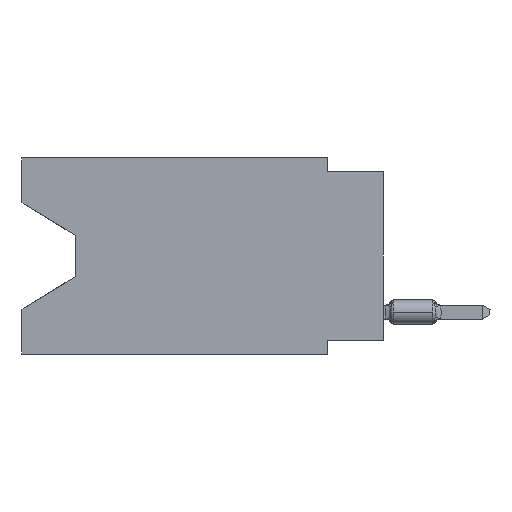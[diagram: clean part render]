
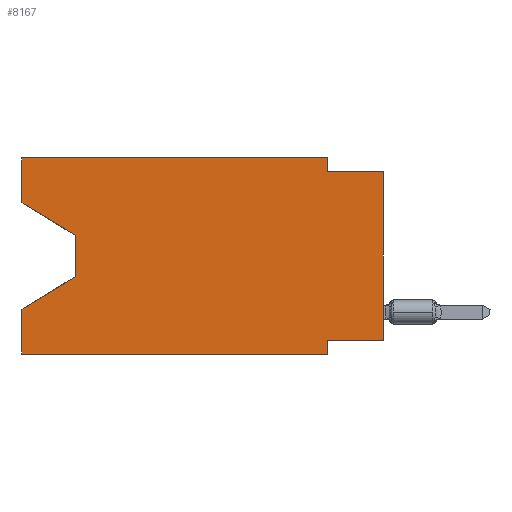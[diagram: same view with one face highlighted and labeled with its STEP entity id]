
A CAD part, left-side view. The second image highlights one B-rep face of the part: STEP entity #8167.
In plain terms, the highlighted planar face has unit normal (-1, 0, 0).
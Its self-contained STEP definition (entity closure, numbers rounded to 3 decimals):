
#788 = DIRECTION ( 'NONE',  ( 0., -1., 0. ) ) ;
#833 = VECTOR ( 'NONE', #54040, 1000. ) ;
#1441 = ORIENTED_EDGE ( 'NONE', *, *, #10999, .F. ) ;
#1702 = ORIENTED_EDGE ( 'NONE', *, *, #21773, .T. ) ;
#2384 = VERTEX_POINT ( 'NONE', #18390 ) ;
#2740 = EDGE_LOOP ( 'NONE', ( #49282, #25133, #4400, #50572, #1702, #9972, #33076, #35058, #36360, #19335, #1441, #18348 ) ) ;
#3293 = VECTOR ( 'NONE', #17079, 1000. ) ;
#3613 = AXIS2_PLACEMENT_3D ( 'NONE', #37514, #12886, #21559 ) ;
#4103 = EDGE_CURVE ( 'NONE', #17922, #8524, #13659, .T. ) ;
#4398 = EDGE_CURVE ( 'NONE', #19168, #21981, #38615, .T. ) ;
#4400 = ORIENTED_EDGE ( 'NONE', *, *, #4398, .T. ) ;
#4711 = LINE ( 'NONE', #21198, #5902 ) ;
#5011 = LINE ( 'NONE', #39121, #32295 ) ;
#5902 = VECTOR ( 'NONE', #788, 1000. ) ;
#5940 = LINE ( 'NONE', #22972, #15642 ) ;
#6770 = DIRECTION ( 'NONE',  ( 0., 0., 1. ) ) ;
#7312 = CARTESIAN_POINT ( 'NONE',  ( 0., 0., -0.635 ) ) ;
#7810 = CARTESIAN_POINT ( 'NONE',  ( 0., 2.54, -8.255 ) ) ;
#7895 = VECTOR ( 'NONE', #50334, 1000. ) ;
#8167 = ADVANCED_FACE ( 'NONE', ( #8705 ), #28830, .F. ) ;
#8524 = VERTEX_POINT ( 'NONE', #7810 ) ;
#8705 = FACE_OUTER_BOUND ( 'NONE', #2740, .T. ) ;
#9911 = DIRECTION ( 'NONE',  ( 0., -1., 0. ) ) ;
#9972 = ORIENTED_EDGE ( 'NONE', *, *, #40160, .F. ) ;
#10999 = EDGE_CURVE ( 'NONE', #2384, #32348, #34797, .T. ) ;
#12886 = DIRECTION ( 'NONE',  ( 1., 0., 0. ) ) ;
#12942 = VECTOR ( 'NONE', #26208, 1000. ) ;
#13306 = VERTEX_POINT ( 'NONE', #50629 ) ;
#13659 = LINE ( 'NONE', #30708, #47019 ) ;
#13821 = CARTESIAN_POINT ( 'NONE',  ( 0., 16.383, 0. ) ) ;
#13863 = VECTOR ( 'NONE', #47947, 1000. ) ;
#14074 = EDGE_CURVE ( 'NONE', #17922, #25388, #25661, .T. ) ;
#14593 = EDGE_CURVE ( 'NONE', #32348, #13306, #22775, .T. ) ;
#15642 = VECTOR ( 'NONE', #6770, 1000. ) ;
#17079 = DIRECTION ( 'NONE',  ( 0., 0.855, -0.519 ) ) ;
#17922 = VERTEX_POINT ( 'NONE', #38385 ) ;
#18348 = ORIENTED_EDGE ( 'NONE', *, *, #31240, .F. ) ;
#18390 = CARTESIAN_POINT ( 'NONE',  ( 0., 16.383, 0. ) ) ;
#19168 = VERTEX_POINT ( 'NONE', #25033 ) ;
#19335 = ORIENTED_EDGE ( 'NONE', *, *, #14593, .F. ) ;
#20267 = VERTEX_POINT ( 'NONE', #33148 ) ;
#20434 = CARTESIAN_POINT ( 'NONE',  ( 0., 16.383, -2.038 ) ) ;
#20675 = VERTEX_POINT ( 'NONE', #20975 ) ;
#20975 = CARTESIAN_POINT ( 'NONE',  ( 0., 13.97, -3.505 ) ) ;
#21198 = CARTESIAN_POINT ( 'NONE',  ( 0., 0., -0.635 ) ) ;
#21559 = DIRECTION ( 'NONE',  ( 0., 0., -1. ) ) ;
#21773 = EDGE_CURVE ( 'NONE', #35954, #21992, #54590, .T. ) ;
#21981 = VERTEX_POINT ( 'NONE', #51226 ) ;
#21992 = VERTEX_POINT ( 'NONE', #52329 ) ;
#22157 = EDGE_CURVE ( 'NONE', #20267, #20675, #33284, .T. ) ;
#22775 = LINE ( 'NONE', #39579, #13863 ) ;
#22972 = CARTESIAN_POINT ( 'NONE',  ( 0., 16.383, 0. ) ) ;
#23643 = EDGE_CURVE ( 'NONE', #20675, #19168, #45393, .T. ) ;
#24403 = DIRECTION ( 'NONE',  ( 0., 0., -1. ) ) ;
#25033 = CARTESIAN_POINT ( 'NONE',  ( 0., 13.97, -5.385 ) ) ;
#25133 = ORIENTED_EDGE ( 'NONE', *, *, #23643, .T. ) ;
#25139 = DIRECTION ( 'NONE',  ( 0., 0., 1. ) ) ;
#25388 = VERTEX_POINT ( 'NONE', #7312 ) ;
#25661 = LINE ( 'NONE', #42734, #12942 ) ;
#26208 = DIRECTION ( 'NONE',  ( 0., 0., 1. ) ) ;
#28039 = VECTOR ( 'NONE', #25139, 1000. ) ;
#28830 = PLANE ( 'NONE',  #3613 ) ;
#28874 = CARTESIAN_POINT ( 'NONE',  ( 0., 16.383, -8.89 ) ) ;
#30708 = CARTESIAN_POINT ( 'NONE',  ( 0., 0., -8.255 ) ) ;
#31240 = EDGE_CURVE ( 'NONE', #20267, #2384, #5940, .T. ) ;
#31466 = VECTOR ( 'NONE', #9911, 1000. ) ;
#32295 = VECTOR ( 'NONE', #34910, 1000. ) ;
#32348 = VERTEX_POINT ( 'NONE', #46680 ) ;
#33076 = ORIENTED_EDGE ( 'NONE', *, *, #4103, .F. ) ;
#33148 = CARTESIAN_POINT ( 'NONE',  ( 0., 16.383, -2.038 ) ) ;
#33284 = LINE ( 'NONE', #20434, #7895 ) ;
#33353 = CARTESIAN_POINT ( 'NONE',  ( 0., 13.97, -3.505 ) ) ;
#34131 = CARTESIAN_POINT ( 'NONE',  ( 0., 13.97, -5.385 ) ) ;
#34797 = LINE ( 'NONE', #13821, #31466 ) ;
#34910 = DIRECTION ( 'NONE',  ( 0., 0., -1. ) ) ;
#35058 = ORIENTED_EDGE ( 'NONE', *, *, #14074, .T. ) ;
#35954 = VERTEX_POINT ( 'NONE', #52363 ) ;
#36360 = ORIENTED_EDGE ( 'NONE', *, *, #53120, .F. ) ;
#37514 = CARTESIAN_POINT ( 'NONE',  ( 0., 16.383, 0. ) ) ;
#38385 = CARTESIAN_POINT ( 'NONE',  ( 0., 0., -8.255 ) ) ;
#38615 = LINE ( 'NONE', #34131, #3293 ) ;
#38851 = CARTESIAN_POINT ( 'NONE',  ( 0., 16.383, 0. ) ) ;
#39121 = CARTESIAN_POINT ( 'NONE',  ( 0., 2.54, -8.89 ) ) ;
#39579 = CARTESIAN_POINT ( 'NONE',  ( 0., 2.54, 0. ) ) ;
#40160 = EDGE_CURVE ( 'NONE', #8524, #21992, #5011, .T. ) ;
#41062 = VECTOR ( 'NONE', #24403, 1000. ) ;
#42734 = CARTESIAN_POINT ( 'NONE',  ( 0., 0., 0. ) ) ;
#43574 = DIRECTION ( 'NONE',  ( 0., 1., 0. ) ) ;
#45393 = LINE ( 'NONE', #33353, #41062 ) ;
#46680 = CARTESIAN_POINT ( 'NONE',  ( 0., 2.54, 0. ) ) ;
#47019 = VECTOR ( 'NONE', #43574, 1000. ) ;
#47947 = DIRECTION ( 'NONE',  ( 0., 0., -1. ) ) ;
#49282 = ORIENTED_EDGE ( 'NONE', *, *, #22157, .T. ) ;
#50334 = DIRECTION ( 'NONE',  ( 0., -0.855, -0.519 ) ) ;
#50572 = ORIENTED_EDGE ( 'NONE', *, *, #51440, .F. ) ;
#50629 = CARTESIAN_POINT ( 'NONE',  ( 0., 2.54, -0.635 ) ) ;
#51139 = LINE ( 'NONE', #38851, #28039 ) ;
#51226 = CARTESIAN_POINT ( 'NONE',  ( 0., 16.383, -6.852 ) ) ;
#51440 = EDGE_CURVE ( 'NONE', #35954, #21981, #51139, .T. ) ;
#52329 = CARTESIAN_POINT ( 'NONE',  ( 0., 2.54, -8.89 ) ) ;
#52363 = CARTESIAN_POINT ( 'NONE',  ( 0., 16.383, -8.89 ) ) ;
#53120 = EDGE_CURVE ( 'NONE', #13306, #25388, #4711, .T. ) ;
#54040 = DIRECTION ( 'NONE',  ( 0., -1., 0. ) ) ;
#54590 = LINE ( 'NONE', #28874, #833 ) ;
